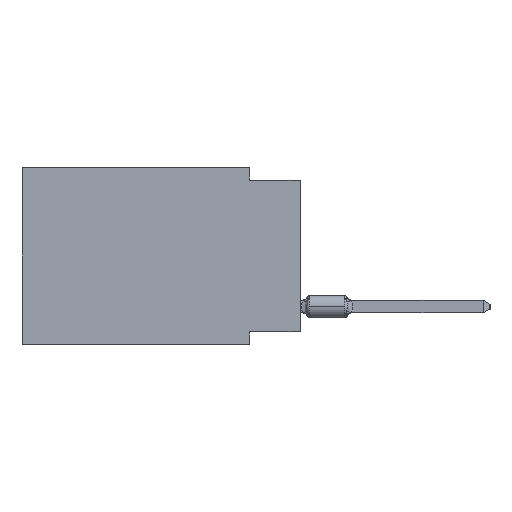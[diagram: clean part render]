
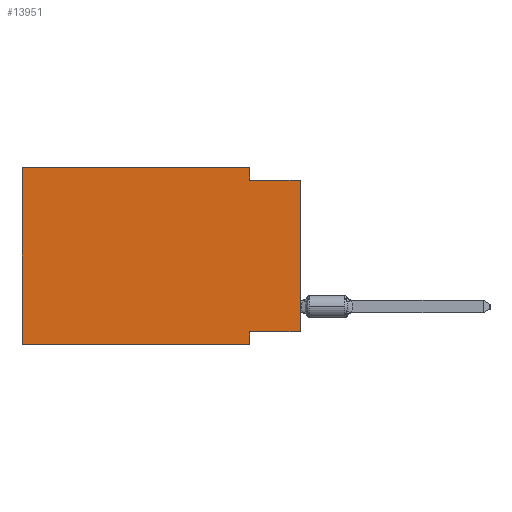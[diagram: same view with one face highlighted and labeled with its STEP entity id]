
A CAD part, left-side view. The second image highlights one B-rep face of the part: STEP entity #13951.
In plain terms, the highlighted planar face has unit normal (-1, 0, 0).
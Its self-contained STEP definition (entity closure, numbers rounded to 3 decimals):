
#167 = CARTESIAN_POINT ( 'NONE',  ( 0., 2.54, -8.89 ) ) ;
#1557 = AXIS2_PLACEMENT_3D ( 'NONE', #44512, #39513, #13060 ) ;
#2131 = EDGE_LOOP ( 'NONE', ( #40687, #48809, #21988, #50086, #31748, #19665, #56860, #46519 ) ) ;
#2326 = VERTEX_POINT ( 'NONE', #48981 ) ;
#3446 = VECTOR ( 'NONE', #26904, 1000. ) ;
#5041 = EDGE_CURVE ( 'NONE', #8417, #37620, #35199, .T. ) ;
#5804 = VERTEX_POINT ( 'NONE', #16796 ) ;
#6933 = VECTOR ( 'NONE', #18056, 1000. ) ;
#8417 = VERTEX_POINT ( 'NONE', #20649 ) ;
#9606 = DIRECTION ( 'NONE',  ( 0., -1., 0. ) ) ;
#11845 = VECTOR ( 'NONE', #25205, 1000. ) ;
#11899 = PLANE ( 'NONE',  #1557 ) ;
#13060 = DIRECTION ( 'NONE',  ( 0., 0., -1. ) ) ;
#13951 = ADVANCED_FACE ( 'NONE', ( #21071 ), #11899, .F. ) ;
#15807 = LINE ( 'NONE', #42530, #40127 ) ;
#16657 = LINE ( 'NONE', #34781, #54621 ) ;
#16796 = CARTESIAN_POINT ( 'NONE',  ( 0., 2.54, 0. ) ) ;
#17169 = CARTESIAN_POINT ( 'NONE',  ( 0., 13.97, 0. ) ) ;
#17348 = CARTESIAN_POINT ( 'NONE',  ( 0., 2.54, -8.255 ) ) ;
#17934 = DIRECTION ( 'NONE',  ( 0., 0., 1. ) ) ;
#17956 = VERTEX_POINT ( 'NONE', #53502 ) ;
#18056 = DIRECTION ( 'NONE',  ( 0., 0., 1. ) ) ;
#19665 = ORIENTED_EDGE ( 'NONE', *, *, #37736, .T. ) ;
#20649 = CARTESIAN_POINT ( 'NONE',  ( 0., 0., -8.255 ) ) ;
#20936 = CARTESIAN_POINT ( 'NONE',  ( 0., 13.97, -8.89 ) ) ;
#20971 = VECTOR ( 'NONE', #17934, 1000. ) ;
#21071 = FACE_OUTER_BOUND ( 'NONE', #2131, .T. ) ;
#21988 = ORIENTED_EDGE ( 'NONE', *, *, #37154, .F. ) ;
#22099 = CARTESIAN_POINT ( 'NONE',  ( 0., 0., 0. ) ) ;
#22182 = VECTOR ( 'NONE', #31991, 1000. ) ;
#23802 = EDGE_CURVE ( 'NONE', #26519, #17956, #48670, .T. ) ;
#23856 = LINE ( 'NONE', #47043, #35637 ) ;
#24115 = CARTESIAN_POINT ( 'NONE',  ( 0., 2.54, -8.89 ) ) ;
#25205 = DIRECTION ( 'NONE',  ( 0., 0., -1. ) ) ;
#26087 = VERTEX_POINT ( 'NONE', #24115 ) ;
#26357 = LINE ( 'NONE', #44445, #11845 ) ;
#26519 = VERTEX_POINT ( 'NONE', #20936 ) ;
#26870 = LINE ( 'NONE', #22099, #20971 ) ;
#26904 = DIRECTION ( 'NONE',  ( 0., 1., 0. ) ) ;
#28076 = EDGE_CURVE ( 'NONE', #2326, #48481, #15807, .T. ) ;
#29456 = DIRECTION ( 'NONE',  ( 0., -1., 0. ) ) ;
#30782 = CARTESIAN_POINT ( 'NONE',  ( 0., 0., -8.255 ) ) ;
#30808 = EDGE_CURVE ( 'NONE', #37620, #26087, #53929, .T. ) ;
#31748 = ORIENTED_EDGE ( 'NONE', *, *, #23802, .F. ) ;
#31991 = DIRECTION ( 'NONE',  ( 0., 0., -1. ) ) ;
#33905 = DIRECTION ( 'NONE',  ( 0., -1., 0. ) ) ;
#34781 = CARTESIAN_POINT ( 'NONE',  ( 0., 13.97, 0. ) ) ;
#35199 = LINE ( 'NONE', #30782, #3446 ) ;
#35637 = VECTOR ( 'NONE', #9606, 1000. ) ;
#37154 = EDGE_CURVE ( 'NONE', #5804, #2326, #26357, .T. ) ;
#37620 = VERTEX_POINT ( 'NONE', #17348 ) ;
#37736 = EDGE_CURVE ( 'NONE', #26519, #26087, #23856, .T. ) ;
#38342 = EDGE_CURVE ( 'NONE', #17956, #5804, #16657, .T. ) ;
#39513 = DIRECTION ( 'NONE',  ( 1., 0., 0. ) ) ;
#40127 = VECTOR ( 'NONE', #29456, 1000. ) ;
#40687 = ORIENTED_EDGE ( 'NONE', *, *, #54421, .T. ) ;
#42530 = CARTESIAN_POINT ( 'NONE',  ( 0., 0., -0.635 ) ) ;
#44445 = CARTESIAN_POINT ( 'NONE',  ( 0., 2.54, 0. ) ) ;
#44512 = CARTESIAN_POINT ( 'NONE',  ( 0., 13.97, 0. ) ) ;
#46519 = ORIENTED_EDGE ( 'NONE', *, *, #5041, .F. ) ;
#47043 = CARTESIAN_POINT ( 'NONE',  ( 0., 13.97, -8.89 ) ) ;
#48481 = VERTEX_POINT ( 'NONE', #48614 ) ;
#48614 = CARTESIAN_POINT ( 'NONE',  ( 0., 0., -0.635 ) ) ;
#48670 = LINE ( 'NONE', #17169, #6933 ) ;
#48809 = ORIENTED_EDGE ( 'NONE', *, *, #28076, .F. ) ;
#48981 = CARTESIAN_POINT ( 'NONE',  ( 0., 2.54, -0.635 ) ) ;
#50086 = ORIENTED_EDGE ( 'NONE', *, *, #38342, .F. ) ;
#53502 = CARTESIAN_POINT ( 'NONE',  ( 0., 13.97, 0. ) ) ;
#53929 = LINE ( 'NONE', #167, #22182 ) ;
#54421 = EDGE_CURVE ( 'NONE', #8417, #48481, #26870, .T. ) ;
#54621 = VECTOR ( 'NONE', #33905, 1000. ) ;
#56860 = ORIENTED_EDGE ( 'NONE', *, *, #30808, .F. ) ;
